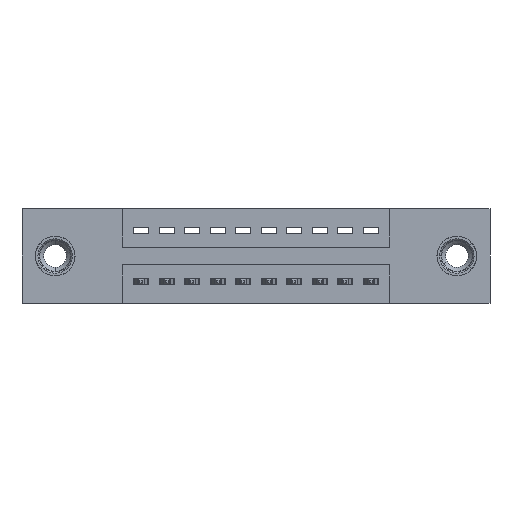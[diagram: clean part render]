
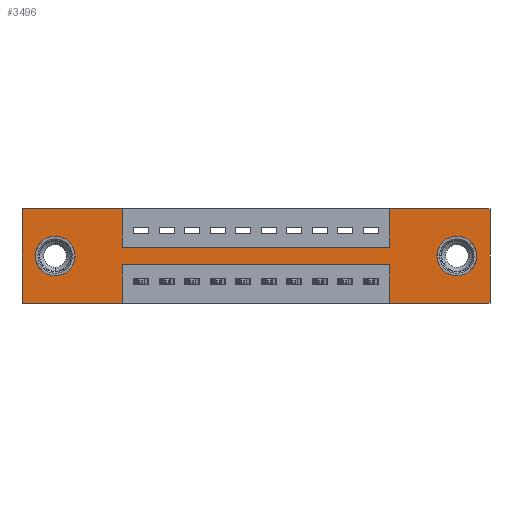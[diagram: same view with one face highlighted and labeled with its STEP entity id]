
A CAD part, front view. The second image highlights one B-rep face of the part: STEP entity #3496.
In plain terms, the highlighted planar face has unit normal (0, -1, 0).
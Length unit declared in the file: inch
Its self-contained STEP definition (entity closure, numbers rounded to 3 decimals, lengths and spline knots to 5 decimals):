
#3 = CARTESIAN_POINT ( 'NONE',  ( 0., 0., -0.37 ) ) ;
#121 = FACE_OUTER_BOUND ( 'NONE', #5542, .T. ) ;
#129 = DIRECTION ( 'NONE',  ( 0., 0., 1. ) ) ;
#134 = VERTEX_POINT ( 'NONE', #8552 ) ;
#144 = VECTOR ( 'NONE', #11791, 39.37008 ) ;
#170 = LINE ( 'NONE', #11545, #7882 ) ;
#367 = ORIENTED_EDGE ( 'NONE', *, *, #11304, .T. ) ;
#408 = EDGE_CURVE ( 'NONE', #134, #1810, #11103, .T. ) ;
#656 = VERTEX_POINT ( 'NONE', #12433 ) ;
#734 = CARTESIAN_POINT ( 'NONE',  ( 1.705, 0., -0.185 ) ) ;
#801 = ORIENTED_EDGE ( 'NONE', *, *, #3868, .T. ) ;
#999 = CARTESIAN_POINT ( 'NONE',  ( 1.4425, 0., -0.15 ) ) ;
#1021 = LINE ( 'NONE', #10134, #12195 ) ;
#1227 = FACE_BOUND ( 'NONE', #7107, .T. ) ;
#1316 = DIRECTION ( 'NONE',  ( 0., 1., 0. ) ) ;
#1399 = CARTESIAN_POINT ( 'NONE',  ( 1.835, 0., -0.37 ) ) ;
#1430 = CARTESIAN_POINT ( 'NONE',  ( 1.835, 0., 0. ) ) ;
#1458 = DIRECTION ( 'NONE',  ( 0., 0., 1. ) ) ;
#1560 = LINE ( 'NONE', #9064, #2668 ) ;
#1650 = AXIS2_PLACEMENT_3D ( 'NONE', #734, #7853, #3856 ) ;
#1810 = VERTEX_POINT ( 'NONE', #11919 ) ;
#1867 = ORIENTED_EDGE ( 'NONE', *, *, #12259, .T. ) ;
#2079 = CARTESIAN_POINT ( 'NONE',  ( 1.4425, 0., 0. ) ) ;
#2082 = LINE ( 'NONE', #3, #12300 ) ;
#2184 = VERTEX_POINT ( 'NONE', #7585 ) ;
#2283 = DIRECTION ( 'NONE',  ( 0., 0., 1. ) ) ;
#2315 = ORIENTED_EDGE ( 'NONE', *, *, #3872, .T. ) ;
#2325 = ORIENTED_EDGE ( 'NONE', *, *, #6201, .F. ) ;
#2573 = ORIENTED_EDGE ( 'NONE', *, *, #4230, .F. ) ;
#2654 = VECTOR ( 'NONE', #8421, 39.37008 ) ;
#2668 = VECTOR ( 'NONE', #5929, 39.37008 ) ;
#2719 = VECTOR ( 'NONE', #10782, 39.37008 ) ;
#2766 = LINE ( 'NONE', #5461, #10510 ) ;
#2824 = PLANE ( 'NONE',  #6896 ) ;
#2865 = DIRECTION ( 'NONE',  ( 0., -1., 0. ) ) ;
#2895 = VERTEX_POINT ( 'NONE', #5528 ) ;
#2958 = VERTEX_POINT ( 'NONE', #5348 ) ;
#2993 = DIRECTION ( 'NONE',  ( 0., 0., -1. ) ) ;
#3188 = DIRECTION ( 'NONE',  ( 0., 0., -1. ) ) ;
#3232 = CARTESIAN_POINT ( 'NONE',  ( 0.13, 0., -0.185 ) ) ;
#3496 = ADVANCED_FACE ( 'NONE', ( #1227, #5449, #121 ), #2824, .T. ) ;
#3814 = VERTEX_POINT ( 'NONE', #1399 ) ;
#3856 = DIRECTION ( 'NONE',  ( 0., 0., -1. ) ) ;
#3859 = DIRECTION ( 'NONE',  ( 0., 0., -1. ) ) ;
#3866 = ORIENTED_EDGE ( 'NONE', *, *, #6066, .F. ) ;
#3868 = EDGE_CURVE ( 'NONE', #7244, #2958, #6388, .T. ) ;
#3872 = EDGE_CURVE ( 'NONE', #2958, #7244, #7925, .T. ) ;
#4005 = VERTEX_POINT ( 'NONE', #11515 ) ;
#4172 = DIRECTION ( 'NONE',  ( 0., 0., 1. ) ) ;
#4230 = EDGE_CURVE ( 'NONE', #8913, #12817, #8070, .T. ) ;
#4387 = CARTESIAN_POINT ( 'NONE',  ( 0.3925, 0., -0.15 ) ) ;
#4458 = EDGE_CURVE ( 'NONE', #5969, #8913, #8058, .T. ) ;
#4484 = VERTEX_POINT ( 'NONE', #4720 ) ;
#4544 = DIRECTION ( 'NONE',  ( 0., 0., 1. ) ) ;
#4597 = ORIENTED_EDGE ( 'NONE', *, *, #6745, .F. ) ;
#4631 = VECTOR ( 'NONE', #3188, 39.37008 ) ;
#4720 = CARTESIAN_POINT ( 'NONE',  ( 0.13, 0., -0.263 ) ) ;
#4794 = EDGE_CURVE ( 'NONE', #5153, #6241, #2082, .T. ) ;
#4958 = EDGE_CURVE ( 'NONE', #2895, #134, #170, .T. ) ;
#5060 = DIRECTION ( 'NONE',  ( -1., 0., 0. ) ) ;
#5153 = VERTEX_POINT ( 'NONE', #10543 ) ;
#5221 = ORIENTED_EDGE ( 'NONE', *, *, #8343, .F. ) ;
#5307 = CARTESIAN_POINT ( 'NONE',  ( 0.13, 0., -0.185 ) ) ;
#5348 = CARTESIAN_POINT ( 'NONE',  ( 1.705, 0., -0.263 ) ) ;
#5449 = FACE_BOUND ( 'NONE', #12649, .T. ) ;
#5461 = CARTESIAN_POINT ( 'NONE',  ( 0., 0., 0. ) ) ;
#5528 = CARTESIAN_POINT ( 'NONE',  ( 1.4425, 0., -0.37 ) ) ;
#5542 = EDGE_LOOP ( 'NONE', ( #5221, #11556, #6172, #2325, #4597, #7149, #9092, #2573, #6045, #3866, #12173, #8004 ) ) ;
#5615 = EDGE_CURVE ( 'NONE', #7362, #4005, #11345, .T. ) ;
#5754 = DIRECTION ( 'NONE',  ( 0., 0., -1. ) ) ;
#5872 = LINE ( 'NONE', #7168, #4631 ) ;
#5929 = DIRECTION ( 'NONE',  ( -1., 0., 0. ) ) ;
#5969 = VERTEX_POINT ( 'NONE', #9632 ) ;
#5975 = CARTESIAN_POINT ( 'NONE',  ( 0., 0., -0.37 ) ) ;
#6043 = AXIS2_PLACEMENT_3D ( 'NONE', #5307, #11299, #4172 ) ;
#6045 = ORIENTED_EDGE ( 'NONE', *, *, #4458, .F. ) ;
#6066 = EDGE_CURVE ( 'NONE', #656, #5969, #11810, .T. ) ;
#6172 = ORIENTED_EDGE ( 'NONE', *, *, #4958, .F. ) ;
#6201 = EDGE_CURVE ( 'NONE', #3814, #2895, #1560, .T. ) ;
#6241 = VERTEX_POINT ( 'NONE', #5975 ) ;
#6352 = CARTESIAN_POINT ( 'NONE',  ( 0., 0., 0. ) ) ;
#6388 = CIRCLE ( 'NONE', #1650, 0.078 ) ;
#6555 = LINE ( 'NONE', #1430, #2654 ) ;
#6745 = EDGE_CURVE ( 'NONE', #4005, #3814, #6555, .T. ) ;
#6896 = AXIS2_PLACEMENT_3D ( 'NONE', #8999, #2865, #2993 ) ;
#7047 = VECTOR ( 'NONE', #11544, 39.37008 ) ;
#7107 = EDGE_LOOP ( 'NONE', ( #801, #2315 ) ) ;
#7149 = ORIENTED_EDGE ( 'NONE', *, *, #5615, .F. ) ;
#7168 = CARTESIAN_POINT ( 'NONE',  ( 0.3925, 0., -0.37 ) ) ;
#7244 = VERTEX_POINT ( 'NONE', #7248 ) ;
#7248 = CARTESIAN_POINT ( 'NONE',  ( 1.705, 0., -0.107 ) ) ;
#7362 = VERTEX_POINT ( 'NONE', #2079 ) ;
#7385 = CARTESIAN_POINT ( 'NONE',  ( 0.3925, 0., -0.22 ) ) ;
#7573 = CARTESIAN_POINT ( 'NONE',  ( 0., 0., 0. ) ) ;
#7585 = CARTESIAN_POINT ( 'NONE',  ( 0.13, 0., -0.107 ) ) ;
#7853 = DIRECTION ( 'NONE',  ( 0., 1., 0. ) ) ;
#7882 = VECTOR ( 'NONE', #1458, 39.37008 ) ;
#7925 = CIRCLE ( 'NONE', #9490, 0.078 ) ;
#8004 = ORIENTED_EDGE ( 'NONE', *, *, #4794, .F. ) ;
#8011 = AXIS2_PLACEMENT_3D ( 'NONE', #3232, #1316, #2283 ) ;
#8058 = LINE ( 'NONE', #10885, #8870 ) ;
#8070 = LINE ( 'NONE', #4387, #2719 ) ;
#8119 = CIRCLE ( 'NONE', #8011, 0.078 ) ;
#8130 = CARTESIAN_POINT ( 'NONE',  ( 0.3925, 0., -0.15 ) ) ;
#8343 = EDGE_CURVE ( 'NONE', #1810, #5153, #5872, .T. ) ;
#8421 = DIRECTION ( 'NONE',  ( 0., 0., -1. ) ) ;
#8552 = CARTESIAN_POINT ( 'NONE',  ( 1.4425, 0., -0.22 ) ) ;
#8605 = EDGE_CURVE ( 'NONE', #6241, #656, #2766, .T. ) ;
#8870 = VECTOR ( 'NONE', #3859, 39.37008 ) ;
#8913 = VERTEX_POINT ( 'NONE', #8130 ) ;
#8999 = CARTESIAN_POINT ( 'NONE',  ( 0., 0., -0.37 ) ) ;
#9064 = CARTESIAN_POINT ( 'NONE',  ( 0., 0., -0.37 ) ) ;
#9092 = ORIENTED_EDGE ( 'NONE', *, *, #11663, .F. ) ;
#9171 = DIRECTION ( 'NONE',  ( -1., 0., 0. ) ) ;
#9490 = AXIS2_PLACEMENT_3D ( 'NONE', #9893, #11826, #5754 ) ;
#9632 = CARTESIAN_POINT ( 'NONE',  ( 0.3925, 0., 0. ) ) ;
#9893 = CARTESIAN_POINT ( 'NONE',  ( 1.705, 0., -0.185 ) ) ;
#10134 = CARTESIAN_POINT ( 'NONE',  ( 1.4425, 0., 0. ) ) ;
#10510 = VECTOR ( 'NONE', #4544, 39.37008 ) ;
#10543 = CARTESIAN_POINT ( 'NONE',  ( 0.3925, 0., -0.37 ) ) ;
#10782 = DIRECTION ( 'NONE',  ( 1., 0., 0. ) ) ;
#10885 = CARTESIAN_POINT ( 'NONE',  ( 0.3925, 0., 0. ) ) ;
#11103 = LINE ( 'NONE', #7385, #11721 ) ;
#11299 = DIRECTION ( 'NONE',  ( 0., 1., 0. ) ) ;
#11304 = EDGE_CURVE ( 'NONE', #2184, #4484, #8119, .T. ) ;
#11345 = LINE ( 'NONE', #6352, #7047 ) ;
#11515 = CARTESIAN_POINT ( 'NONE',  ( 1.835, 0., 0. ) ) ;
#11544 = DIRECTION ( 'NONE',  ( 1., 0., 0. ) ) ;
#11545 = CARTESIAN_POINT ( 'NONE',  ( 1.4425, 0., -0.37 ) ) ;
#11556 = ORIENTED_EDGE ( 'NONE', *, *, #408, .F. ) ;
#11663 = EDGE_CURVE ( 'NONE', #12817, #7362, #1021, .T. ) ;
#11721 = VECTOR ( 'NONE', #5060, 39.37008 ) ;
#11791 = DIRECTION ( 'NONE',  ( 1., 0., 0. ) ) ;
#11810 = LINE ( 'NONE', #7573, #144 ) ;
#11826 = DIRECTION ( 'NONE',  ( 0., 1., 0. ) ) ;
#11919 = CARTESIAN_POINT ( 'NONE',  ( 0.3925, 0., -0.22 ) ) ;
#12173 = ORIENTED_EDGE ( 'NONE', *, *, #8605, .F. ) ;
#12195 = VECTOR ( 'NONE', #129, 39.37008 ) ;
#12259 = EDGE_CURVE ( 'NONE', #4484, #2184, #12335, .T. ) ;
#12300 = VECTOR ( 'NONE', #9171, 39.37008 ) ;
#12335 = CIRCLE ( 'NONE', #6043, 0.078 ) ;
#12433 = CARTESIAN_POINT ( 'NONE',  ( 0., 0., 0. ) ) ;
#12649 = EDGE_LOOP ( 'NONE', ( #367, #1867 ) ) ;
#12817 = VERTEX_POINT ( 'NONE', #999 ) ;
